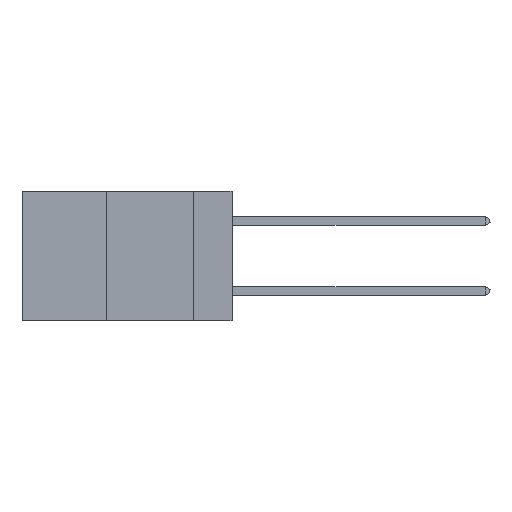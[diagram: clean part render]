
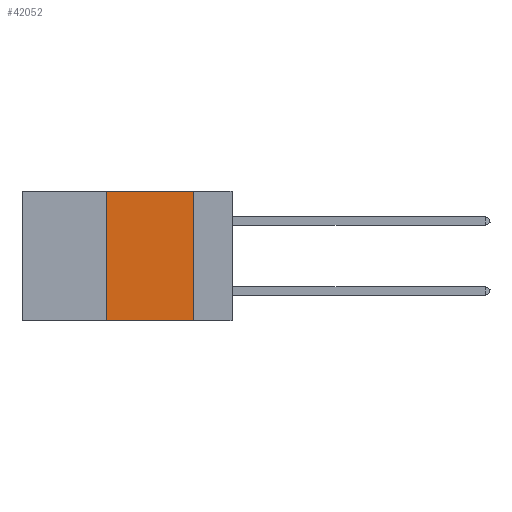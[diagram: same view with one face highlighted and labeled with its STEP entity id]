
A CAD part, left-side view. The second image highlights one B-rep face of the part: STEP entity #42052.
In plain terms, the highlighted planar face has unit normal (-1, 0, 0).
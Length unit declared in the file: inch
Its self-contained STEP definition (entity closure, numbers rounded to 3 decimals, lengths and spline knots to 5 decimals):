
#4301 = EDGE_CURVE ( 'NONE', #25210, #8056, #5536, .T. ) ;
#5536 = LINE ( 'NONE', #36777, #41605 ) ;
#5576 = EDGE_CURVE ( 'NONE', #25210, #23810, #19852, .T. ) ;
#7829 = AXIS2_PLACEMENT_3D ( 'NONE', #38531, #10768, #35258 ) ;
#8056 = VERTEX_POINT ( 'NONE', #40915 ) ;
#9831 = FACE_OUTER_BOUND ( 'NONE', #42687, .T. ) ;
#10768 = DIRECTION ( 'NONE',  ( 1., 0., 0. ) ) ;
#11561 = VECTOR ( 'NONE', #18465, 39.37008 ) ;
#13103 = VECTOR ( 'NONE', #29322, 39.37008 ) ;
#14225 = LINE ( 'NONE', #36274, #13103 ) ;
#14692 = DIRECTION ( 'NONE',  ( 0., 0., -1. ) ) ;
#16055 = ORIENTED_EDGE ( 'NONE', *, *, #32633, .F. ) ;
#16405 = CARTESIAN_POINT ( 'NONE',  ( 0., 0.36, 0. ) ) ;
#18062 = CARTESIAN_POINT ( 'NONE',  ( 0., 0.11, 0. ) ) ;
#18465 = DIRECTION ( 'NONE',  ( 0., 0., 1. ) ) ;
#19852 = LINE ( 'NONE', #39175, #11561 ) ;
#19931 = EDGE_CURVE ( 'NONE', #24286, #8056, #21915, .T. ) ;
#21915 = LINE ( 'NONE', #18062, #38153 ) ;
#22983 = DIRECTION ( 'NONE',  ( 0., -1., 0. ) ) ;
#23810 = VERTEX_POINT ( 'NONE', #16405 ) ;
#24286 = VERTEX_POINT ( 'NONE', #34194 ) ;
#25210 = VERTEX_POINT ( 'NONE', #35182 ) ;
#26046 = ORIENTED_EDGE ( 'NONE', *, *, #4301, .T. ) ;
#29322 = DIRECTION ( 'NONE',  ( 0., -1., 0. ) ) ;
#31796 = PLANE ( 'NONE',  #7829 ) ;
#32633 = EDGE_CURVE ( 'NONE', #23810, #24286, #14225, .T. ) ;
#34194 = CARTESIAN_POINT ( 'NONE',  ( 0., 0.11, 0. ) ) ;
#35182 = CARTESIAN_POINT ( 'NONE',  ( 0., 0.36, -0.37 ) ) ;
#35258 = DIRECTION ( 'NONE',  ( 0., 0., -1. ) ) ;
#36274 = CARTESIAN_POINT ( 'NONE',  ( 0., 0.6, 0. ) ) ;
#36777 = CARTESIAN_POINT ( 'NONE',  ( 0., 0.6, -0.37 ) ) ;
#38153 = VECTOR ( 'NONE', #14692, 39.37008 ) ;
#38531 = CARTESIAN_POINT ( 'NONE',  ( 0., 0.6, 0. ) ) ;
#39175 = CARTESIAN_POINT ( 'NONE',  ( 0., 0.36, 0. ) ) ;
#39550 = ORIENTED_EDGE ( 'NONE', *, *, #19931, .F. ) ;
#40915 = CARTESIAN_POINT ( 'NONE',  ( 0., 0.11, -0.37 ) ) ;
#41605 = VECTOR ( 'NONE', #22983, 39.37008 ) ;
#42052 = ADVANCED_FACE ( 'NONE', ( #9831 ), #31796, .F. ) ;
#42687 = EDGE_LOOP ( 'NONE', ( #39550, #16055, #44571, #26046 ) ) ;
#44571 = ORIENTED_EDGE ( 'NONE', *, *, #5576, .F. ) ;
